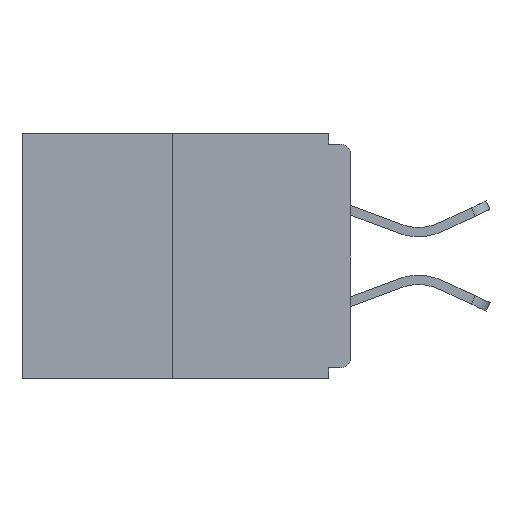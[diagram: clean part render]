
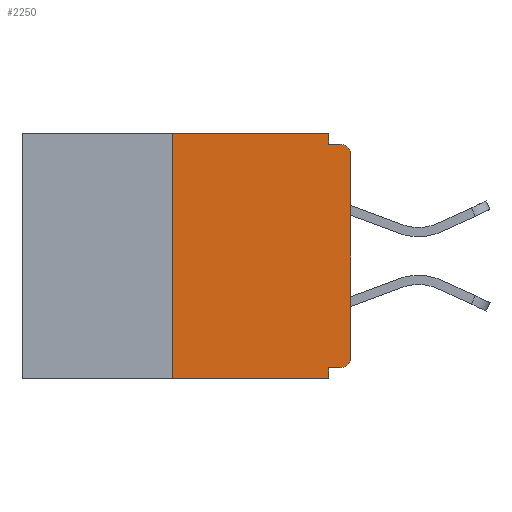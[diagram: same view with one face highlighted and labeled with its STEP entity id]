
A CAD part, left-side view. The second image highlights one B-rep face of the part: STEP entity #2250.
In plain terms, the highlighted planar face has unit normal (-1, 0, 0).
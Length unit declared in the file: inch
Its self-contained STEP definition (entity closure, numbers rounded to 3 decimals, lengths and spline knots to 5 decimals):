
#428 = VECTOR ( 'NONE', #484, 39.37008 ) ;
#484 = DIRECTION ( 'NONE',  ( 0., -1., 0. ) ) ;
#489 = VECTOR ( 'NONE', #9066, 39.37008 ) ;
#634 = LINE ( 'NONE', #18953, #8133 ) ;
#1075 = EDGE_CURVE ( 'NONE', #14035, #20818, #18199, .T. ) ;
#1152 = DIRECTION ( 'NONE',  ( 0., 0., -1. ) ) ;
#1478 = EDGE_CURVE ( 'NONE', #20818, #2555, #20397, .T. ) ;
#1619 = DIRECTION ( 'NONE',  ( 1., 0., 0. ) ) ;
#1654 = VERTEX_POINT ( 'NONE', #16634 ) ;
#1772 = LINE ( 'NONE', #23044, #12025 ) ;
#1850 = CARTESIAN_POINT ( 'NONE',  ( 0., 0.031, -0.343 ) ) ;
#2130 = EDGE_CURVE ( 'NONE', #17817, #15803, #634, .T. ) ;
#2250 = ADVANCED_FACE ( 'NONE', ( #11473 ), #3512, .F. ) ;
#2266 = ORIENTED_EDGE ( 'NONE', *, *, #18361, .F. ) ;
#2555 = VERTEX_POINT ( 'NONE', #6836 ) ;
#2742 = VERTEX_POINT ( 'NONE', #22338 ) ;
#2905 = AXIS2_PLACEMENT_3D ( 'NONE', #22452, #10069, #1152 ) ;
#3291 = CARTESIAN_POINT ( 'NONE',  ( 0., 0.46, 0. ) ) ;
#3512 = PLANE ( 'NONE',  #17022 ) ;
#3537 = ORIENTED_EDGE ( 'NONE', *, *, #14801, .F. ) ;
#3710 = CARTESIAN_POINT ( 'NONE',  ( 0., 0., -0.015 ) ) ;
#4095 = ORIENTED_EDGE ( 'NONE', *, *, #14678, .F. ) ;
#4349 = LINE ( 'NONE', #19982, #428 ) ;
#4957 = CARTESIAN_POINT ( 'NONE',  ( 0., 0.015, -0.328 ) ) ;
#5112 = VECTOR ( 'NONE', #13356, 39.37008 ) ;
#5272 = VERTEX_POINT ( 'NONE', #20477 ) ;
#5959 = LINE ( 'NONE', #3710, #22393 ) ;
#6345 = DIRECTION ( 'NONE',  ( 0., 0., -1. ) ) ;
#6697 = DIRECTION ( 'NONE',  ( 0., 0., -1. ) ) ;
#6836 = CARTESIAN_POINT ( 'NONE',  ( 0., 0., -0.03 ) ) ;
#6988 = DIRECTION ( 'NONE',  ( 0., 0., -1. ) ) ;
#7054 = CARTESIAN_POINT ( 'NONE',  ( 0., 0., -0.328 ) ) ;
#7158 = VECTOR ( 'NONE', #8977, 39.37008 ) ;
#8049 = DIRECTION ( 'NONE',  ( -1., 0., 0. ) ) ;
#8133 = VECTOR ( 'NONE', #15350, 39.37008 ) ;
#8351 = EDGE_CURVE ( 'NONE', #15581, #15803, #9801, .T. ) ;
#8429 = CARTESIAN_POINT ( 'NONE',  ( 0., 0.25, -0.343 ) ) ;
#8885 = ORIENTED_EDGE ( 'NONE', *, *, #2130, .F. ) ;
#8977 = DIRECTION ( 'NONE',  ( 0., 0., 1. ) ) ;
#9066 = DIRECTION ( 'NONE',  ( 0., 1., 0. ) ) ;
#9759 = ORIENTED_EDGE ( 'NONE', *, *, #22399, .F. ) ;
#9801 = LINE ( 'NONE', #20294, #5112 ) ;
#10069 = DIRECTION ( 'NONE',  ( -1., 0., 0. ) ) ;
#10493 = LINE ( 'NONE', #21492, #7158 ) ;
#10899 = DIRECTION ( 'NONE',  ( 0., -1., 0. ) ) ;
#11473 = FACE_OUTER_BOUND ( 'NONE', #12500, .T. ) ;
#11821 = CIRCLE ( 'NONE', #18369, 0.015 ) ;
#12025 = VECTOR ( 'NONE', #6697, 39.37008 ) ;
#12176 = EDGE_CURVE ( 'NONE', #15581, #1654, #10493, .T. ) ;
#12232 = DIRECTION ( 'NONE',  ( 0., 0., 1. ) ) ;
#12500 = EDGE_LOOP ( 'NONE', ( #9759, #21811, #21002, #8885, #2266, #17792, #18386, #21162, #4095, #3537 ) ) ;
#13356 = DIRECTION ( 'NONE',  ( 0., -1., 0. ) ) ;
#14035 = VERTEX_POINT ( 'NONE', #4957 ) ;
#14678 = EDGE_CURVE ( 'NONE', #14714, #5272, #5959, .T. ) ;
#14714 = VERTEX_POINT ( 'NONE', #15447 ) ;
#14801 = EDGE_CURVE ( 'NONE', #2742, #14714, #1772, .T. ) ;
#15056 = CARTESIAN_POINT ( 'NONE',  ( 0., 0., -0.313 ) ) ;
#15069 = VECTOR ( 'NONE', #12232, 39.37008 ) ;
#15350 = DIRECTION ( 'NONE',  ( 0., 0., -1. ) ) ;
#15447 = CARTESIAN_POINT ( 'NONE',  ( 0., 0.031, -0.015 ) ) ;
#15581 = VERTEX_POINT ( 'NONE', #8429 ) ;
#15803 = VERTEX_POINT ( 'NONE', #1850 ) ;
#16634 = CARTESIAN_POINT ( 'NONE',  ( 0., 0.25, 0. ) ) ;
#16973 = CARTESIAN_POINT ( 'NONE',  ( 0., 0.015, -0.03 ) ) ;
#17022 = AXIS2_PLACEMENT_3D ( 'NONE', #3291, #1619, #6988 ) ;
#17792 = ORIENTED_EDGE ( 'NONE', *, *, #1075, .T. ) ;
#17817 = VERTEX_POINT ( 'NONE', #18647 ) ;
#18199 = CIRCLE ( 'NONE', #2905, 0.015 ) ;
#18361 = EDGE_CURVE ( 'NONE', #14035, #17817, #21347, .T. ) ;
#18369 = AXIS2_PLACEMENT_3D ( 'NONE', #16973, #8049, #6345 ) ;
#18386 = ORIENTED_EDGE ( 'NONE', *, *, #1478, .T. ) ;
#18647 = CARTESIAN_POINT ( 'NONE',  ( 0., 0.031, -0.328 ) ) ;
#18953 = CARTESIAN_POINT ( 'NONE',  ( 0., 0.031, -0.343 ) ) ;
#19471 = CARTESIAN_POINT ( 'NONE',  ( 0., 0., 0. ) ) ;
#19982 = CARTESIAN_POINT ( 'NONE',  ( 0., 0.46, 0. ) ) ;
#20294 = CARTESIAN_POINT ( 'NONE',  ( 0., 0.46, -0.343 ) ) ;
#20397 = LINE ( 'NONE', #19471, #15069 ) ;
#20477 = CARTESIAN_POINT ( 'NONE',  ( 0., 0.015, -0.015 ) ) ;
#20818 = VERTEX_POINT ( 'NONE', #15056 ) ;
#21002 = ORIENTED_EDGE ( 'NONE', *, *, #8351, .T. ) ;
#21162 = ORIENTED_EDGE ( 'NONE', *, *, #21432, .T. ) ;
#21347 = LINE ( 'NONE', #7054, #489 ) ;
#21432 = EDGE_CURVE ( 'NONE', #2555, #5272, #11821, .T. ) ;
#21492 = CARTESIAN_POINT ( 'NONE',  ( 0., 0.25, 0. ) ) ;
#21811 = ORIENTED_EDGE ( 'NONE', *, *, #12176, .F. ) ;
#22338 = CARTESIAN_POINT ( 'NONE',  ( 0., 0.031, 0. ) ) ;
#22393 = VECTOR ( 'NONE', #10899, 39.37008 ) ;
#22399 = EDGE_CURVE ( 'NONE', #1654, #2742, #4349, .T. ) ;
#22452 = CARTESIAN_POINT ( 'NONE',  ( 0., 0.015, -0.313 ) ) ;
#23044 = CARTESIAN_POINT ( 'NONE',  ( 0., 0.031, 0. ) ) ;
